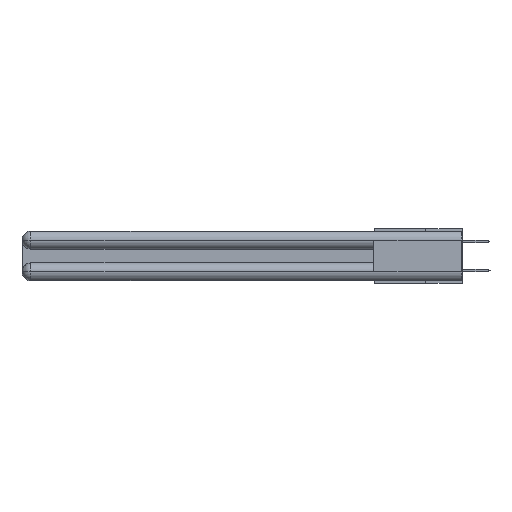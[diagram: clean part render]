
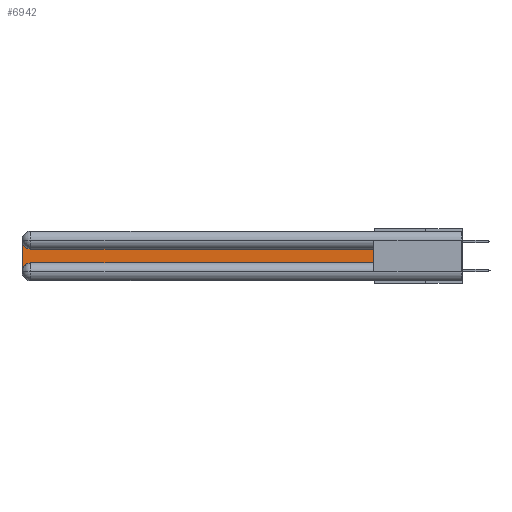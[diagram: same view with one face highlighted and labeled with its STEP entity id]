
A CAD part, left-side view. The second image highlights one B-rep face of the part: STEP entity #6942.
In plain terms, the highlighted planar face has unit normal (-1, 0, 0).
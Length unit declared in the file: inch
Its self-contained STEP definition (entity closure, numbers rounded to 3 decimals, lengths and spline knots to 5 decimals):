
#1478 = VERTEX_POINT ( 'NONE', #21011 ) ;
#1532 = VERTEX_POINT ( 'NONE', #6076 ) ;
#1957 = EDGE_LOOP ( 'NONE', ( #12731, #28597, #23432, #15649, #10839, #25211 ) ) ;
#2343 = FACE_OUTER_BOUND ( 'NONE', #1957, .T. ) ;
#2700 = VECTOR ( 'NONE', #18976, 39.37008 ) ;
#2808 = VECTOR ( 'NONE', #22780, 39.37008 ) ;
#4382 = DIRECTION ( 'NONE',  ( 1., 0., 0. ) ) ;
#5024 = EDGE_CURVE ( 'NONE', #12168, #1532, #5243, .T. ) ;
#5219 = CARTESIAN_POINT ( 'NONE',  ( 0.075, 2.94, -0.2775 ) ) ;
#5243 = LINE ( 'NONE', #21320, #2808 ) ;
#6076 = CARTESIAN_POINT ( 'NONE',  ( 0.075, 3., -0.2775 ) ) ;
#6626 = VERTEX_POINT ( 'NONE', #12040 ) ;
#6942 = ADVANCED_FACE ( 'NONE', ( #2343 ), #22673, .F. ) ;
#7242 = DIRECTION ( 'NONE',  ( 0., 0., -1. ) ) ;
#7657 = AXIS2_PLACEMENT_3D ( 'NONE', #5219, #16375, #16267 ) ;
#9476 = DIRECTION ( 'NONE',  ( 0., -1., 0. ) ) ;
#10111 = VERTEX_POINT ( 'NONE', #26738 ) ;
#10839 = ORIENTED_EDGE ( 'NONE', *, *, #16467, .T. ) ;
#10869 = DIRECTION ( 'NONE',  ( 0., 0., 1. ) ) ;
#10963 = CIRCLE ( 'NONE', #7657, 0.06 ) ;
#11470 = EDGE_CURVE ( 'NONE', #16003, #1478, #12443, .T. ) ;
#12040 = CARTESIAN_POINT ( 'NONE',  ( 0.075, 2.94, -0.2175 ) ) ;
#12078 = CARTESIAN_POINT ( 'NONE',  ( 0.075, 0.6, -0.1225 ) ) ;
#12168 = VERTEX_POINT ( 'NONE', #12986 ) ;
#12442 = LINE ( 'NONE', #20522, #23276 ) ;
#12443 = LINE ( 'NONE', #12078, #2700 ) ;
#12706 = CARTESIAN_POINT ( 'NONE',  ( 0.075, 0.6, -0.1225 ) ) ;
#12731 = ORIENTED_EDGE ( 'NONE', *, *, #11470, .T. ) ;
#12771 = EDGE_CURVE ( 'NONE', #1532, #6626, #10963, .T. ) ;
#12986 = CARTESIAN_POINT ( 'NONE',  ( 0.075, 3., -0.0625 ) ) ;
#13429 = EDGE_CURVE ( 'NONE', #10111, #16003, #26697, .T. ) ;
#15649 = ORIENTED_EDGE ( 'NONE', *, *, #12771, .T. ) ;
#16003 = VERTEX_POINT ( 'NONE', #12706 ) ;
#16267 = DIRECTION ( 'NONE',  ( 0., 0., -1. ) ) ;
#16277 = EDGE_CURVE ( 'NONE', #1478, #12168, #28564, .T. ) ;
#16375 = DIRECTION ( 'NONE',  ( 1., 0., 0. ) ) ;
#16467 = EDGE_CURVE ( 'NONE', #6626, #10111, #12442, .T. ) ;
#18455 = CARTESIAN_POINT ( 'NONE',  ( 0.075, 3., -0.1225 ) ) ;
#18976 = DIRECTION ( 'NONE',  ( 0., 1., 0. ) ) ;
#20160 = CARTESIAN_POINT ( 'NONE',  ( 0.075, 2.94, -0.0625 ) ) ;
#20522 = CARTESIAN_POINT ( 'NONE',  ( 0.075, 0.6, -0.2175 ) ) ;
#21011 = CARTESIAN_POINT ( 'NONE',  ( 0.075, 2.94, -0.1225 ) ) ;
#21320 = CARTESIAN_POINT ( 'NONE',  ( 0.075, 3., -0.2175 ) ) ;
#22117 = AXIS2_PLACEMENT_3D ( 'NONE', #20160, #4382, #24755 ) ;
#22673 = PLANE ( 'NONE',  #27594 ) ;
#22780 = DIRECTION ( 'NONE',  ( 0., 0., -1. ) ) ;
#23046 = DIRECTION ( 'NONE',  ( 1., 0., 0. ) ) ;
#23276 = VECTOR ( 'NONE', #9476, 39.37008 ) ;
#23432 = ORIENTED_EDGE ( 'NONE', *, *, #5024, .T. ) ;
#24755 = DIRECTION ( 'NONE',  ( 0., 0., -1. ) ) ;
#25211 = ORIENTED_EDGE ( 'NONE', *, *, #13429, .T. ) ;
#25293 = VECTOR ( 'NONE', #10869, 39.37008 ) ;
#26697 = LINE ( 'NONE', #28872, #25293 ) ;
#26738 = CARTESIAN_POINT ( 'NONE',  ( 0.075, 0.6, -0.2175 ) ) ;
#27594 = AXIS2_PLACEMENT_3D ( 'NONE', #18455, #23046, #7242 ) ;
#28564 = CIRCLE ( 'NONE', #22117, 0.06 ) ;
#28597 = ORIENTED_EDGE ( 'NONE', *, *, #16277, .T. ) ;
#28872 = CARTESIAN_POINT ( 'NONE',  ( 0.075, 0.6, -0.2175 ) ) ;
